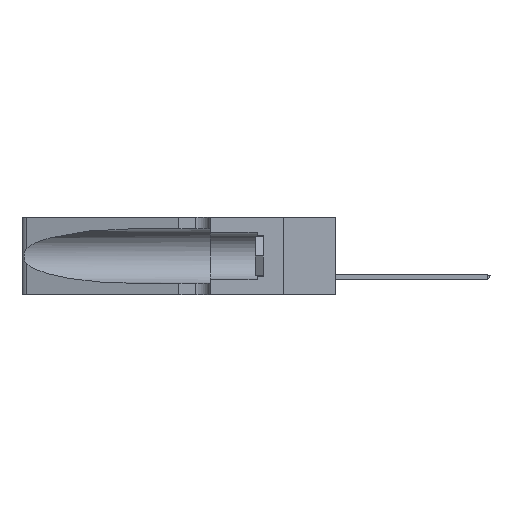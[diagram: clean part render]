
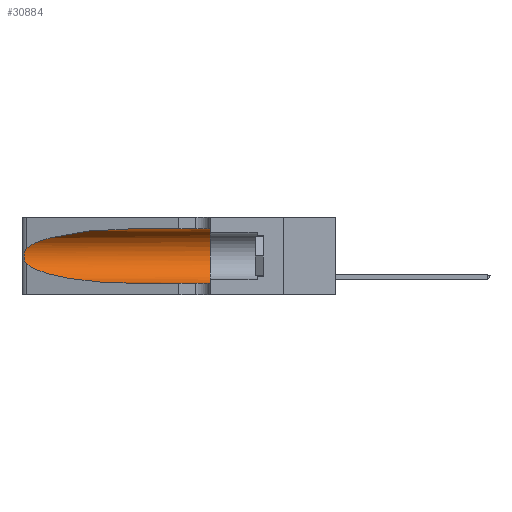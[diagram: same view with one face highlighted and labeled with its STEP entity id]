
A CAD part, left-side view. The second image highlights one B-rep face of the part: STEP entity #30884.
In plain terms, the highlighted cylindrical face has radius 3.308 mm (diameter 6.617 mm), a partial arc.
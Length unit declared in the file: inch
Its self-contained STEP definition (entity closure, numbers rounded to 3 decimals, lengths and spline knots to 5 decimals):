
#36 = AXIS2_PLACEMENT_3D ( 'NONE', #13398, #36386, #24622 ) ;
#720 = ORIENTED_EDGE ( 'NONE', *, *, #15419, .T. ) ;
#1039 = VERTEX_POINT ( 'NONE', #26748 ) ;
#1756 = CARTESIAN_POINT ( 'NONE',  ( 0.1305, 0.35, 0.05475 ) ) ;
#1968 = VERTEX_POINT ( 'NONE', #7966 ) ;
#2058 = CARTESIAN_POINT ( 'NONE',  ( 0.25854, 1.2359, 0.20912 ) ) ;
#2648 = CIRCLE ( 'NONE', #36, 0.13025 ) ;
#3972 = VERTEX_POINT ( 'NONE', #1756 ) ;
#4126 =( BOUNDED_CURVE ( )  B_SPLINE_CURVE ( 3, ( #27894, #10671, #36685, #34991 ),
 .UNSPECIFIED., .F., .T. ) 
 B_SPLINE_CURVE_WITH_KNOTS ( ( 4, 4 ),
 ( 1.5708, 2.84003 ),
 .UNSPECIFIED. ) 
 CURVE ( )  GEOMETRIC_REPRESENTATION_ITEM ( )  RATIONAL_B_SPLINE_CURVE ( ( 1., 0.87, 0.87, 1. ) ) 
 REPRESENTATION_ITEM ( '' )  );
#5295 = CARTESIAN_POINT ( 'NONE',  ( 0.26075, 1.23896, 0.178 ) ) ;
#5626 = EDGE_CURVE ( 'NONE', #9760, #3972, #2648, .T. ) ;
#6150 = EDGE_LOOP ( 'NONE', ( #8613, #34484, #720, #34347, #18120, #22564 ) ) ;
#7300 = CARTESIAN_POINT ( 'NONE',  ( 0.25487, 1.22718, 0.14631 ) ) ;
#7966 = CARTESIAN_POINT ( 'NONE',  ( 0.1305, 0.72297, 0.31525 ) ) ;
#8494 = VECTOR ( 'NONE', #15652, 39.37008 ) ;
#8613 = ORIENTED_EDGE ( 'NONE', *, *, #18459, .T. ) ;
#9760 = VERTEX_POINT ( 'NONE', #23311 ) ;
#9819 = CARTESIAN_POINT ( 'NONE',  ( 0.1305, 1.61858, 0.31525 ) ) ;
#10671 = CARTESIAN_POINT ( 'NONE',  ( 0.18966, 0.96281, 0.31525 ) ) ;
#10766 = CARTESIAN_POINT ( 'NONE',  ( 0.25856, 1.23593, 0.16098 ) ) ;
#11511 = EDGE_CURVE ( 'NONE', #24595, #1039, #35979, .T. ) ;
#13398 = CARTESIAN_POINT ( 'NONE',  ( 0.1305, 0.35, 0.185 ) ) ;
#14018 = CARTESIAN_POINT ( 'NONE',  ( 0.25487, 1.22718, 0.22369 ) ) ;
#15419 = EDGE_CURVE ( 'NONE', #1039, #37048, #35257, .T. ) ;
#15652 = DIRECTION ( 'NONE',  ( 0., -1., 0. ) ) ;
#15917 = CARTESIAN_POINT ( 'NONE',  ( 0.2373, 1.15595, 0.08982 ) ) ;
#18111 = EDGE_CURVE ( 'NONE', #37048, #3972, #34768, .T. ) ;
#18120 = ORIENTED_EDGE ( 'NONE', *, *, #5626, .F. ) ;
#18387 = LINE ( 'NONE', #9819, #8494 ) ;
#18459 = EDGE_CURVE ( 'NONE', #1968, #24595, #4126, .T. ) ;
#18612 = CARTESIAN_POINT ( 'NONE',  ( 0.25639, 1.23184, 0.21858 ) ) ;
#19066 = CARTESIAN_POINT ( 'NONE',  ( 0.1305, 1.61858, 0.05475 ) ) ;
#21195 = CYLINDRICAL_SURFACE ( 'NONE', #35203, 0.13025 ) ;
#21668 = CARTESIAN_POINT ( 'NONE',  ( 0.18966, 0.96281, 0.05475 ) ) ;
#22215 = CARTESIAN_POINT ( 'NONE',  ( 0.26018, 1.23835, 0.19895 ) ) ;
#22468 = CARTESIAN_POINT ( 'NONE',  ( 0.26017, 1.23833, 0.17102 ) ) ;
#22564 = ORIENTED_EDGE ( 'NONE', *, *, #25258, .F. ) ;
#22638 = DIRECTION ( 'NONE',  ( 0., -1., 0. ) ) ;
#23311 = CARTESIAN_POINT ( 'NONE',  ( 0.1305, 0.35, 0.31525 ) ) ;
#24595 = VERTEX_POINT ( 'NONE', #14018 ) ;
#24600 = CARTESIAN_POINT ( 'NONE',  ( 0.1305, 0.72297, 0.05475 ) ) ;
#24622 = DIRECTION ( 'NONE',  ( 0., 0., 1. ) ) ;
#25258 = EDGE_CURVE ( 'NONE', #1968, #9760, #18387, .T. ) ;
#25498 = CARTESIAN_POINT ( 'NONE',  ( 0.25789, 1.23486, 0.15765 ) ) ;
#26035 = CARTESIAN_POINT ( 'NONE',  ( 0.25555, 1.22994, 0.2215 ) ) ;
#26493 = DIRECTION ( 'NONE',  ( 0., 0., -1. ) ) ;
#26748 = CARTESIAN_POINT ( 'NONE',  ( 0.25487, 1.22718, 0.14631 ) ) ;
#27187 = VECTOR ( 'NONE', #36174, 39.37008 ) ;
#27685 = CARTESIAN_POINT ( 'NONE',  ( 0.25487, 1.22718, 0.22369 ) ) ;
#27752 = CARTESIAN_POINT ( 'NONE',  ( 0.26075, 1.23896, 0.19203 ) ) ;
#27894 = CARTESIAN_POINT ( 'NONE',  ( 0.1305, 0.72297, 0.31525 ) ) ;
#30096 = CARTESIAN_POINT ( 'NONE',  ( 0.25787, 1.23484, 0.2124 ) ) ;
#30884 = ADVANCED_FACE ( 'NONE', ( #36958 ), #21195, .F. ) ;
#31104 = CARTESIAN_POINT ( 'NONE',  ( 0.25639, 1.23186, 0.15144 ) ) ;
#33211 = CARTESIAN_POINT ( 'NONE',  ( 0.1305, 0.72297, 0.05475 ) ) ;
#33877 = CARTESIAN_POINT ( 'NONE',  ( 0.25555, 1.22993, 0.14849 ) ) ;
#34347 = ORIENTED_EDGE ( 'NONE', *, *, #18111, .T. ) ;
#34410 = CARTESIAN_POINT ( 'NONE',  ( 0.1305, 1.61858, 0.185 ) ) ;
#34484 = ORIENTED_EDGE ( 'NONE', *, *, #11511, .T. ) ;
#34768 = LINE ( 'NONE', #19066, #27187 ) ;
#34991 = CARTESIAN_POINT ( 'NONE',  ( 0.25487, 1.22718, 0.22369 ) ) ;
#35203 = AXIS2_PLACEMENT_3D ( 'NONE', #34410, #22638, #26493 ) ;
#35257 =( BOUNDED_CURVE ( )  B_SPLINE_CURVE ( 3, ( #7300, #15917, #21668, #24600 ),
 .UNSPECIFIED., .F., .F. ) 
 B_SPLINE_CURVE_WITH_KNOTS ( ( 4, 4 ),
 ( 3.44316, 4.71239 ),
 .UNSPECIFIED. ) 
 CURVE ( )  GEOMETRIC_REPRESENTATION_ITEM ( )  RATIONAL_B_SPLINE_CURVE ( ( 1., 0.87, 0.87, 1. ) ) 
 REPRESENTATION_ITEM ( '' )  );
#35979 = B_SPLINE_CURVE_WITH_KNOTS ( 'NONE', 3,
 ( #27685, #26035, #18612, #30096, #2058, #22215, #27752, #5295, #22468, #10766, #25498, #31104, #33877, #36532 ),
 .UNSPECIFIED., .F., .F.,
 ( 4, 2, 2, 2, 2, 2, 4 ),
 ( 0., 0.00027, 0.00053, 0.00107, 0.0016, 0.00187, 0.00214 ),
 .UNSPECIFIED. ) ;
#36174 = DIRECTION ( 'NONE',  ( 0., -1., 0. ) ) ;
#36386 = DIRECTION ( 'NONE',  ( 0., 1., 0. ) ) ;
#36532 = CARTESIAN_POINT ( 'NONE',  ( 0.25487, 1.22718, 0.14631 ) ) ;
#36685 = CARTESIAN_POINT ( 'NONE',  ( 0.2373, 1.15595, 0.28018 ) ) ;
#36958 = FACE_OUTER_BOUND ( 'NONE', #6150, .T. ) ;
#37048 = VERTEX_POINT ( 'NONE', #33211 ) ;
